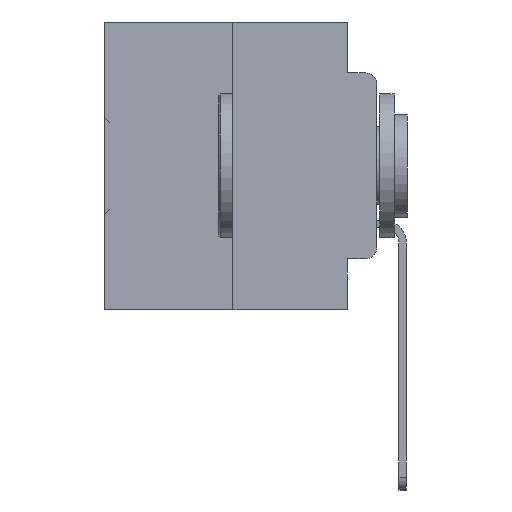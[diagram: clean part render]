
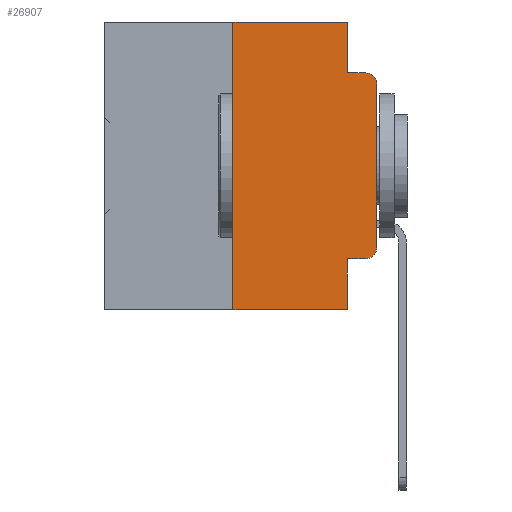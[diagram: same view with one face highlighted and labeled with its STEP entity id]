
A CAD part, left-side view. The second image highlights one B-rep face of the part: STEP entity #26907.
In plain terms, the highlighted planar face has unit normal (-1, 0, 0).
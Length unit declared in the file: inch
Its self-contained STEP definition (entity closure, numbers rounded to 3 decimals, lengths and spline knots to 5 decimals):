
#470 = CARTESIAN_POINT ( 'NONE',  ( 0., 0.02, -0.3915 ) ) ;
#613 = VECTOR ( 'NONE', #5588, 39.37008 ) ;
#686 = VERTEX_POINT ( 'NONE', #35198 ) ;
#1094 = DIRECTION ( 'NONE',  ( 0., -1., 0. ) ) ;
#1345 = EDGE_CURVE ( 'NONE', #29717, #2391, #27174, .T. ) ;
#1527 = EDGE_CURVE ( 'NONE', #6058, #3584, #21693, .T. ) ;
#1631 = CARTESIAN_POINT ( 'NONE',  ( 0., 0., -0.3915 ) ) ;
#2391 = VERTEX_POINT ( 'NONE', #14965 ) ;
#2486 = PLANE ( 'NONE',  #23431 ) ;
#2553 = CARTESIAN_POINT ( 'NONE',  ( 0., 0.051, -0.0885 ) ) ;
#2670 = DIRECTION ( 'NONE',  ( 0., 0., 1. ) ) ;
#2794 = CARTESIAN_POINT ( 'NONE',  ( 0., 0.051, -0.5 ) ) ;
#3503 = DIRECTION ( 'NONE',  ( 0., 0., -1. ) ) ;
#3542 = EDGE_CURVE ( 'NONE', #24863, #29717, #19284, .T. ) ;
#3584 = VERTEX_POINT ( 'NONE', #2794 ) ;
#4838 = VERTEX_POINT ( 'NONE', #9266 ) ;
#5111 = DIRECTION ( 'NONE',  ( 0., 0., -1. ) ) ;
#5588 = DIRECTION ( 'NONE',  ( 0., -1., 0. ) ) ;
#6058 = VERTEX_POINT ( 'NONE', #32359 ) ;
#6089 = VECTOR ( 'NONE', #19619, 39.37008 ) ;
#6970 = DIRECTION ( 'NONE',  ( -1., 0., 0. ) ) ;
#8118 = CARTESIAN_POINT ( 'NONE',  ( 0., 0.051, 0. ) ) ;
#9266 = CARTESIAN_POINT ( 'NONE',  ( 0., 0., -0.1085 ) ) ;
#10551 = AXIS2_PLACEMENT_3D ( 'NONE', #24502, #6970, #27440 ) ;
#11460 = DIRECTION ( 'NONE',  ( 0., 0., -1. ) ) ;
#11468 = VECTOR ( 'NONE', #2670, 39.37008 ) ;
#11485 = VECTOR ( 'NONE', #33435, 39.37008 ) ;
#11530 = EDGE_CURVE ( 'NONE', #2391, #686, #30061, .T. ) ;
#11580 = DIRECTION ( 'NONE',  ( 0., -1., 0. ) ) ;
#11626 = VECTOR ( 'NONE', #11580, 39.37008 ) ;
#12413 = LINE ( 'NONE', #27789, #11485 ) ;
#12861 = CARTESIAN_POINT ( 'NONE',  ( 0., 0.25, -0.5 ) ) ;
#14965 = CARTESIAN_POINT ( 'NONE',  ( 0., 0.051, 0. ) ) ;
#17239 = EDGE_CURVE ( 'NONE', #24863, #3584, #12413, .T. ) ;
#17511 = CARTESIAN_POINT ( 'NONE',  ( 0., 0.051, -0.4115 ) ) ;
#18650 = EDGE_LOOP ( 'NONE', ( #21019, #21481, #22123, #22238, #22617, #22742, #22919, #23265, #23337, #23734 ) ) ;
#19284 = LINE ( 'NONE', #31901, #11468 ) ;
#19445 = LINE ( 'NONE', #17511, #11626 ) ;
#19619 = DIRECTION ( 'NONE',  ( 0., 0., -1. ) ) ;
#21019 = ORIENTED_EDGE ( 'NONE', *, *, #34932, .T. ) ;
#21175 = DIRECTION ( 'NONE',  ( -1., 0., 0. ) ) ;
#21481 = ORIENTED_EDGE ( 'NONE', *, *, #31052, .T. ) ;
#21693 = LINE ( 'NONE', #34034, #6089 ) ;
#21765 = CARTESIAN_POINT ( 'NONE',  ( 0., 0.473, 0. ) ) ;
#22038 = LINE ( 'NONE', #24566, #36523 ) ;
#22123 = ORIENTED_EDGE ( 'NONE', *, *, #25230, .F. ) ;
#22238 = ORIENTED_EDGE ( 'NONE', *, *, #11530, .F. ) ;
#22617 = ORIENTED_EDGE ( 'NONE', *, *, #1345, .F. ) ;
#22742 = ORIENTED_EDGE ( 'NONE', *, *, #3542, .F. ) ;
#22919 = ORIENTED_EDGE ( 'NONE', *, *, #17239, .T. ) ;
#23265 = ORIENTED_EDGE ( 'NONE', *, *, #1527, .F. ) ;
#23337 = ORIENTED_EDGE ( 'NONE', *, *, #33693, .T. ) ;
#23431 = AXIS2_PLACEMENT_3D ( 'NONE', #26035, #28946, #11460 ) ;
#23456 = CARTESIAN_POINT ( 'NONE',  ( 0., 0.25, 0. ) ) ;
#23691 = CARTESIAN_POINT ( 'NONE',  ( 0., 0.02, -0.4115 ) ) ;
#23734 = ORIENTED_EDGE ( 'NONE', *, *, #29828, .T. ) ;
#24151 = LINE ( 'NONE', #2553, #613 ) ;
#24502 = CARTESIAN_POINT ( 'NONE',  ( 0., 0.02, -0.1085 ) ) ;
#24566 = CARTESIAN_POINT ( 'NONE',  ( 0., 0., 0. ) ) ;
#24863 = VERTEX_POINT ( 'NONE', #12861 ) ;
#25230 = EDGE_CURVE ( 'NONE', #686, #30624, #24151, .T. ) ;
#25957 = AXIS2_PLACEMENT_3D ( 'NONE', #470, #21175, #3503 ) ;
#26035 = CARTESIAN_POINT ( 'NONE',  ( 0., 0.473, 0. ) ) ;
#26907 = ADVANCED_FACE ( 'NONE', ( #34431 ), #2486, .F. ) ;
#27174 = LINE ( 'NONE', #21765, #34863 ) ;
#27364 = VERTEX_POINT ( 'NONE', #1631 ) ;
#27440 = DIRECTION ( 'NONE',  ( 0., 0., -1. ) ) ;
#27493 = DIRECTION ( 'NONE',  ( 0., 0., 1. ) ) ;
#27789 = CARTESIAN_POINT ( 'NONE',  ( 0., 0.473, -0.5 ) ) ;
#27849 = CARTESIAN_POINT ( 'NONE',  ( 0., 0.02, -0.0885 ) ) ;
#28946 = DIRECTION ( 'NONE',  ( 1., 0., 0. ) ) ;
#29175 = VECTOR ( 'NONE', #5111, 39.37008 ) ;
#29717 = VERTEX_POINT ( 'NONE', #23456 ) ;
#29828 = EDGE_CURVE ( 'NONE', #36398, #27364, #34638, .T. ) ;
#30061 = LINE ( 'NONE', #8118, #29175 ) ;
#30472 = CIRCLE ( 'NONE', #10551, 0.02 ) ;
#30624 = VERTEX_POINT ( 'NONE', #27849 ) ;
#31052 = EDGE_CURVE ( 'NONE', #4838, #30624, #30472, .T. ) ;
#31901 = CARTESIAN_POINT ( 'NONE',  ( 0., 0.25, 0. ) ) ;
#32359 = CARTESIAN_POINT ( 'NONE',  ( 0., 0.051, -0.4115 ) ) ;
#33435 = DIRECTION ( 'NONE',  ( 0., -1., 0. ) ) ;
#33693 = EDGE_CURVE ( 'NONE', #6058, #36398, #19445, .T. ) ;
#34034 = CARTESIAN_POINT ( 'NONE',  ( 0., 0.051, 0. ) ) ;
#34431 = FACE_OUTER_BOUND ( 'NONE', #18650, .T. ) ;
#34638 = CIRCLE ( 'NONE', #25957, 0.02 ) ;
#34863 = VECTOR ( 'NONE', #1094, 39.37008 ) ;
#34932 = EDGE_CURVE ( 'NONE', #27364, #4838, #22038, .T. ) ;
#35198 = CARTESIAN_POINT ( 'NONE',  ( 0., 0.051, -0.0885 ) ) ;
#36398 = VERTEX_POINT ( 'NONE', #23691 ) ;
#36523 = VECTOR ( 'NONE', #27493, 39.37008 ) ;
